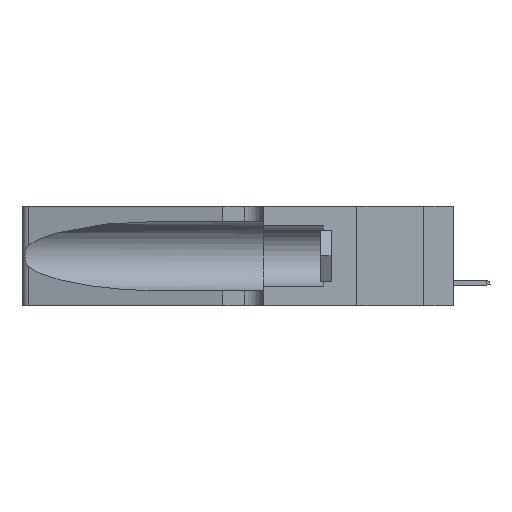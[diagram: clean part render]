
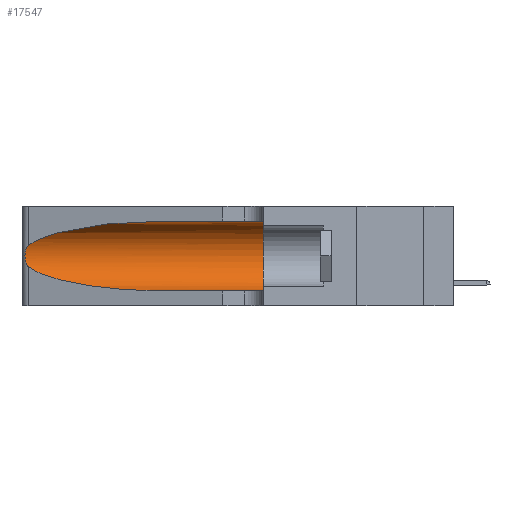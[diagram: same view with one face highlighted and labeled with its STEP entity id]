
A CAD part, left-side view. The second image highlights one B-rep face of the part: STEP entity #17547.
In plain terms, the highlighted cylindrical face has radius 3.308 mm (diameter 6.617 mm), a partial arc.
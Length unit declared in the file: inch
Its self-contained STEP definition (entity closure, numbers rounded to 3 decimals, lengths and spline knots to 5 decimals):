
#443 = VERTEX_POINT ( 'NONE', #13735 ) ;
#626 = CARTESIAN_POINT ( 'NONE',  ( 0.25555, 1.22994, 0.2215 ) ) ;
#1058 = ORIENTED_EDGE ( 'NONE', *, *, #6691, .F. ) ;
#1088 = LINE ( 'NONE', #3801, #13156 ) ;
#1974 = CARTESIAN_POINT ( 'NONE',  ( 0.25487, 1.22718, 0.22369 ) ) ;
#2072 = CARTESIAN_POINT ( 'NONE',  ( 0.26075, 1.23896, 0.178 ) ) ;
#2180 = CYLINDRICAL_SURFACE ( 'NONE', #9871, 0.13025 ) ;
#2988 = CARTESIAN_POINT ( 'NONE',  ( 0.1305, 0.72297, 0.31525 ) ) ;
#3033 = CARTESIAN_POINT ( 'NONE',  ( 0.25487, 1.22718, 0.14631 ) ) ;
#3546 = CARTESIAN_POINT ( 'NONE',  ( 0.26017, 1.23833, 0.17102 ) ) ;
#3664 = VERTEX_POINT ( 'NONE', #7928 ) ;
#3801 = CARTESIAN_POINT ( 'NONE',  ( 0.1305, 1.61858, 0.05475 ) ) ;
#3872 = CARTESIAN_POINT ( 'NONE',  ( 0.1305, 0.72297, 0.05475 ) ) ;
#3875 = DIRECTION ( 'NONE',  ( 0., 0., 1. ) ) ;
#4335 =( BOUNDED_CURVE ( )  B_SPLINE_CURVE ( 3, ( #5751, #5848, #7404, #14877 ),
 .UNSPECIFIED., .F., .F. ) 
 B_SPLINE_CURVE_WITH_KNOTS ( ( 4, 4 ),
 ( 3.44316, 4.71239 ),
 .UNSPECIFIED. ) 
 CURVE ( )  GEOMETRIC_REPRESENTATION_ITEM ( )  RATIONAL_B_SPLINE_CURVE ( ( 1., 0.87, 0.87, 1. ) ) 
 REPRESENTATION_ITEM ( '' )  );
#5751 = CARTESIAN_POINT ( 'NONE',  ( 0.25487, 1.22718, 0.14631 ) ) ;
#5848 = CARTESIAN_POINT ( 'NONE',  ( 0.2373, 1.15595, 0.08982 ) ) ;
#6274 = CARTESIAN_POINT ( 'NONE',  ( 0.25789, 1.23486, 0.15765 ) ) ;
#6386 = DIRECTION ( 'NONE',  ( 0., -1., 0. ) ) ;
#6467 = CARTESIAN_POINT ( 'NONE',  ( 0.26075, 1.23896, 0.19203 ) ) ;
#6649 = CIRCLE ( 'NONE', #16246, 0.13025 ) ;
#6691 = EDGE_CURVE ( 'NONE', #3664, #17697, #8955, .T. ) ;
#6803 = CARTESIAN_POINT ( 'NONE',  ( 0.1305, 0.35, 0.185 ) ) ;
#6945 = CARTESIAN_POINT ( 'NONE',  ( 0.1305, 1.61858, 0.31525 ) ) ;
#7121 = DIRECTION ( 'NONE',  ( 0., -1., 0. ) ) ;
#7404 = CARTESIAN_POINT ( 'NONE',  ( 0.18966, 0.96281, 0.05475 ) ) ;
#7928 = CARTESIAN_POINT ( 'NONE',  ( 0.1305, 0.72297, 0.31525 ) ) ;
#8128 = CARTESIAN_POINT ( 'NONE',  ( 0.25639, 1.23184, 0.21858 ) ) ;
#8182 = DIRECTION ( 'NONE',  ( 0., 1., 0. ) ) ;
#8955 = LINE ( 'NONE', #6945, #16120 ) ;
#9278 = CARTESIAN_POINT ( 'NONE',  ( 0.25487, 1.22718, 0.22369 ) ) ;
#9383 = CARTESIAN_POINT ( 'NONE',  ( 0.25787, 1.23484, 0.2124 ) ) ;
#9396 = FACE_OUTER_BOUND ( 'NONE', #10086, .T. ) ;
#9871 = AXIS2_PLACEMENT_3D ( 'NONE', #12426, #6386, #15494 ) ;
#10086 = EDGE_LOOP ( 'NONE', ( #19157, #13878, #10396, #13663, #14455, #1058 ) ) ;
#10396 = ORIENTED_EDGE ( 'NONE', *, *, #12513, .T. ) ;
#10492 = EDGE_CURVE ( 'NONE', #17967, #16606, #11155, .T. ) ;
#10582 = CARTESIAN_POINT ( 'NONE',  ( 0.18966, 0.96281, 0.31525 ) ) ;
#10850 = CARTESIAN_POINT ( 'NONE',  ( 0.26018, 1.23835, 0.19895 ) ) ;
#10945 = CARTESIAN_POINT ( 'NONE',  ( 0.25639, 1.23186, 0.15144 ) ) ;
#11131 = CARTESIAN_POINT ( 'NONE',  ( 0.25487, 1.22718, 0.14631 ) ) ;
#11155 = B_SPLINE_CURVE_WITH_KNOTS ( 'NONE', 3,
 ( #1974, #626, #8128, #9383, #12232, #10850, #6467, #2072, #3546, #12324, #6274, #10945, #18447, #11131 ),
 .UNSPECIFIED., .F., .F.,
 ( 4, 2, 2, 2, 2, 2, 4 ),
 ( 0., 0.00027, 0.00053, 0.00107, 0.0016, 0.00187, 0.00214 ),
 .UNSPECIFIED. ) ;
#11514 = VERTEX_POINT ( 'NONE', #3872 ) ;
#12232 = CARTESIAN_POINT ( 'NONE',  ( 0.25854, 1.2359, 0.20912 ) ) ;
#12324 = CARTESIAN_POINT ( 'NONE',  ( 0.25856, 1.23593, 0.16098 ) ) ;
#12381 = EDGE_CURVE ( 'NONE', #11514, #443, #1088, .T. ) ;
#12426 = CARTESIAN_POINT ( 'NONE',  ( 0.1305, 1.61858, 0.185 ) ) ;
#12513 = EDGE_CURVE ( 'NONE', #16606, #11514, #4335, .T. ) ;
#12796 = EDGE_CURVE ( 'NONE', #17697, #443, #6649, .T. ) ;
#13156 = VECTOR ( 'NONE', #7121, 39.37008 ) ;
#13663 = ORIENTED_EDGE ( 'NONE', *, *, #12381, .T. ) ;
#13735 = CARTESIAN_POINT ( 'NONE',  ( 0.1305, 0.35, 0.05475 ) ) ;
#13878 = ORIENTED_EDGE ( 'NONE', *, *, #10492, .T. ) ;
#14330 = CARTESIAN_POINT ( 'NONE',  ( 0.1305, 0.35, 0.31525 ) ) ;
#14455 = ORIENTED_EDGE ( 'NONE', *, *, #12796, .F. ) ;
#14747 =( BOUNDED_CURVE ( )  B_SPLINE_CURVE ( 3, ( #2988, #10582, #16463, #15035 ),
 .UNSPECIFIED., .F., .T. ) 
 B_SPLINE_CURVE_WITH_KNOTS ( ( 4, 4 ),
 ( 1.5708, 2.84003 ),
 .UNSPECIFIED. ) 
 CURVE ( )  GEOMETRIC_REPRESENTATION_ITEM ( )  RATIONAL_B_SPLINE_CURVE ( ( 1., 0.87, 0.87, 1. ) ) 
 REPRESENTATION_ITEM ( '' )  );
#14865 = DIRECTION ( 'NONE',  ( 0., -1., 0. ) ) ;
#14877 = CARTESIAN_POINT ( 'NONE',  ( 0.1305, 0.72297, 0.05475 ) ) ;
#15035 = CARTESIAN_POINT ( 'NONE',  ( 0.25487, 1.22718, 0.22369 ) ) ;
#15494 = DIRECTION ( 'NONE',  ( 0., 0., -1. ) ) ;
#16120 = VECTOR ( 'NONE', #14865, 39.37008 ) ;
#16246 = AXIS2_PLACEMENT_3D ( 'NONE', #6803, #8182, #3875 ) ;
#16463 = CARTESIAN_POINT ( 'NONE',  ( 0.2373, 1.15595, 0.28018 ) ) ;
#16606 = VERTEX_POINT ( 'NONE', #3033 ) ;
#17353 = EDGE_CURVE ( 'NONE', #3664, #17967, #14747, .T. ) ;
#17547 = ADVANCED_FACE ( 'NONE', ( #9396 ), #2180, .F. ) ;
#17697 = VERTEX_POINT ( 'NONE', #14330 ) ;
#17967 = VERTEX_POINT ( 'NONE', #9278 ) ;
#18447 = CARTESIAN_POINT ( 'NONE',  ( 0.25555, 1.22993, 0.14849 ) ) ;
#19157 = ORIENTED_EDGE ( 'NONE', *, *, #17353, .T. ) ;
